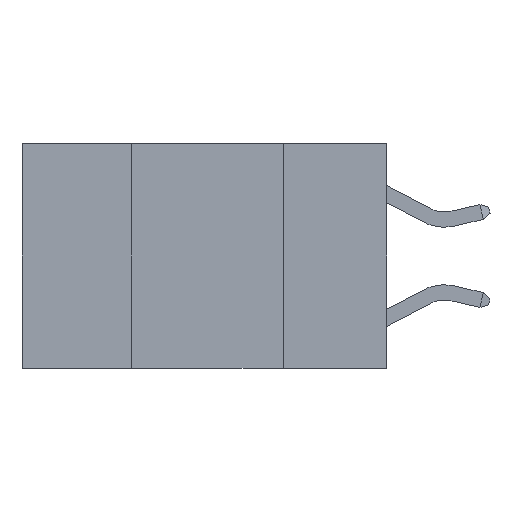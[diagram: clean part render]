
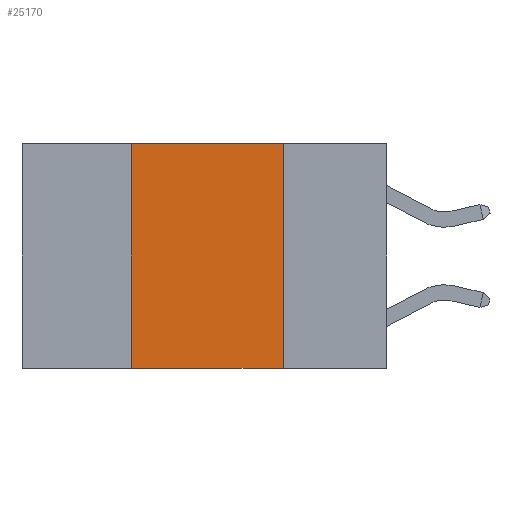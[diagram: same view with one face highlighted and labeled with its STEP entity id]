
A CAD part, left-side view. The second image highlights one B-rep face of the part: STEP entity #25170.
In plain terms, the highlighted planar face has unit normal (-1, 0, 0).
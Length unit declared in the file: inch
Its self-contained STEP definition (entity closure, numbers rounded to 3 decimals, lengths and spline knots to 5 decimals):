
#163 = EDGE_CURVE ( 'NONE', #15536, #4576, #24826, .T. ) ;
#2787 = DIRECTION ( 'NONE',  ( 0., -1., 0. ) ) ;
#3763 = VECTOR ( 'NONE', #21870, 39.37008 ) ;
#4279 = ORIENTED_EDGE ( 'NONE', *, *, #13196, .T. ) ;
#4576 = VERTEX_POINT ( 'NONE', #24128 ) ;
#4646 = DIRECTION ( 'NONE',  ( 0., 0., -1. ) ) ;
#4825 = VERTEX_POINT ( 'NONE', #18416 ) ;
#5744 = AXIS2_PLACEMENT_3D ( 'NONE', #17939, #18027, #4646 ) ;
#6194 = CARTESIAN_POINT ( 'NONE',  ( 0., 0.17, 0. ) ) ;
#6270 = CARTESIAN_POINT ( 'NONE',  ( 0., 0.17, 0. ) ) ;
#6970 = FACE_OUTER_BOUND ( 'NONE', #17908, .T. ) ;
#9546 = CARTESIAN_POINT ( 'NONE',  ( 0., 0.6, -0.37 ) ) ;
#10939 = VECTOR ( 'NONE', #2787, 39.37008 ) ;
#12394 = VECTOR ( 'NONE', #19621, 39.37008 ) ;
#12532 = EDGE_CURVE ( 'NONE', #15535, #15536, #17918, .T. ) ;
#13196 = EDGE_CURVE ( 'NONE', #4825, #4576, #16842, .T. ) ;
#14268 = DIRECTION ( 'NONE',  ( 0., -1., 0. ) ) ;
#15535 = VERTEX_POINT ( 'NONE', #19559 ) ;
#15536 = VERTEX_POINT ( 'NONE', #6194 ) ;
#15578 = EDGE_CURVE ( 'NONE', #4825, #15535, #15699, .T. ) ;
#15699 = LINE ( 'NONE', #19654, #3763 ) ;
#16842 = LINE ( 'NONE', #9546, #10939 ) ;
#17908 = EDGE_LOOP ( 'NONE', ( #26885, #28269, #25866, #4279 ) ) ;
#17918 = LINE ( 'NONE', #25280, #28939 ) ;
#17939 = CARTESIAN_POINT ( 'NONE',  ( 0., 0.6, 0. ) ) ;
#18027 = DIRECTION ( 'NONE',  ( 1., 0., 0. ) ) ;
#18416 = CARTESIAN_POINT ( 'NONE',  ( 0., 0.42, -0.37 ) ) ;
#19559 = CARTESIAN_POINT ( 'NONE',  ( 0., 0.42, 0. ) ) ;
#19621 = DIRECTION ( 'NONE',  ( 0., 0., -1. ) ) ;
#19654 = CARTESIAN_POINT ( 'NONE',  ( 0., 0.42, 0. ) ) ;
#21870 = DIRECTION ( 'NONE',  ( 0., 0., 1. ) ) ;
#24128 = CARTESIAN_POINT ( 'NONE',  ( 0., 0.17, -0.37 ) ) ;
#24826 = LINE ( 'NONE', #6270, #12394 ) ;
#25170 = ADVANCED_FACE ( 'NONE', ( #6970 ), #26802, .F. ) ;
#25280 = CARTESIAN_POINT ( 'NONE',  ( 0., 0.6, 0. ) ) ;
#25866 = ORIENTED_EDGE ( 'NONE', *, *, #15578, .F. ) ;
#26802 = PLANE ( 'NONE',  #5744 ) ;
#26885 = ORIENTED_EDGE ( 'NONE', *, *, #163, .F. ) ;
#28269 = ORIENTED_EDGE ( 'NONE', *, *, #12532, .F. ) ;
#28939 = VECTOR ( 'NONE', #14268, 39.37008 ) ;
